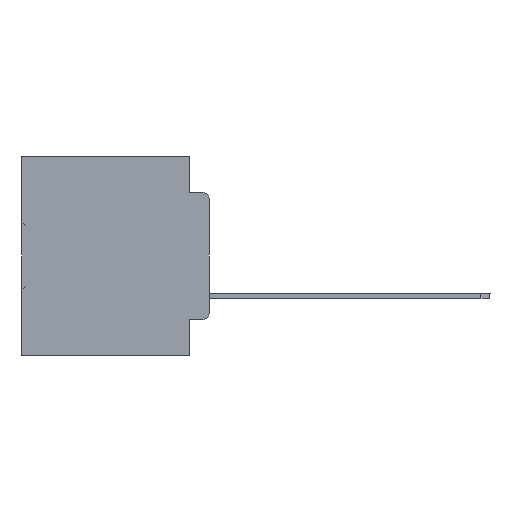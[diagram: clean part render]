
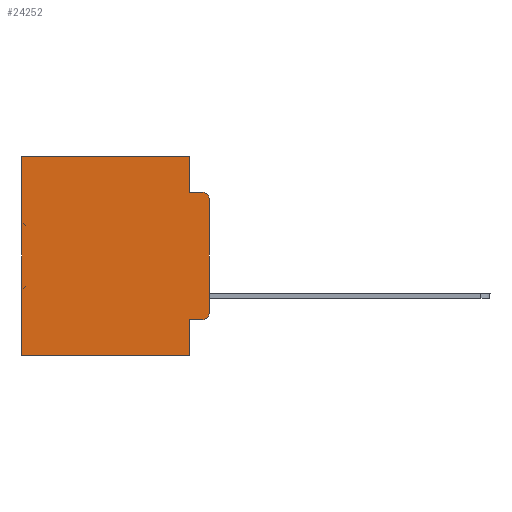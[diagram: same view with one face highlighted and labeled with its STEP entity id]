
A CAD part, left-side view. The second image highlights one B-rep face of the part: STEP entity #24252.
In plain terms, the highlighted planar face has unit normal (-1, 0, 0).
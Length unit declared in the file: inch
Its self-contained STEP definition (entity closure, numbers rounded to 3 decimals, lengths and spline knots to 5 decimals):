
#265 = DIRECTION ( 'NONE',  ( 0., 0., -1. ) ) ;
#486 = DIRECTION ( 'NONE',  ( 0., 1., 0. ) ) ;
#992 = ORIENTED_EDGE ( 'NONE', *, *, #2277, .T. ) ;
#1150 = CARTESIAN_POINT ( 'NONE',  ( 0.298, 0.02, -0.4115 ) ) ;
#1247 = CARTESIAN_POINT ( 'NONE',  ( 0.298, 0., -0.5 ) ) ;
#1260 = EDGE_CURVE ( 'NONE', #4417, #13636, #15243, .T. ) ;
#1427 = CARTESIAN_POINT ( 'NONE',  ( 0.298, 0.051, 0. ) ) ;
#1604 = ORIENTED_EDGE ( 'NONE', *, *, #29339, .F. ) ;
#1828 = ORIENTED_EDGE ( 'NONE', *, *, #32957, .T. ) ;
#1943 = CARTESIAN_POINT ( 'NONE',  ( 0.298, 0., -0.3915 ) ) ;
#2215 = CIRCLE ( 'NONE', #25763, 0.02 ) ;
#2277 = EDGE_CURVE ( 'NONE', #29301, #34442, #7477, .T. ) ;
#2846 = LINE ( 'NONE', #14070, #20878 ) ;
#3327 = CARTESIAN_POINT ( 'NONE',  ( 0.298, 0.051, -0.4115 ) ) ;
#3336 = DIRECTION ( 'NONE',  ( 0., 0., -1. ) ) ;
#3627 = VECTOR ( 'NONE', #486, 39.37008 ) ;
#4417 = VERTEX_POINT ( 'NONE', #9358 ) ;
#4768 = EDGE_CURVE ( 'NONE', #9812, #14329, #6210, .T. ) ;
#5054 = CARTESIAN_POINT ( 'NONE',  ( 0.298, 0.473, 0. ) ) ;
#6210 = LINE ( 'NONE', #36431, #3627 ) ;
#6419 = CARTESIAN_POINT ( 'NONE',  ( 0.298, 0.02, -0.0885 ) ) ;
#6586 = DIRECTION ( 'NONE',  ( 0., 0., -1. ) ) ;
#7319 = VERTEX_POINT ( 'NONE', #1943 ) ;
#7477 = CIRCLE ( 'NONE', #28071, 0.02 ) ;
#8354 = LINE ( 'NONE', #5054, #28795 ) ;
#9358 = CARTESIAN_POINT ( 'NONE',  ( 0.298, 0.051, -0.5 ) ) ;
#9449 = ORIENTED_EDGE ( 'NONE', *, *, #22322, .T. ) ;
#9744 = VECTOR ( 'NONE', #19666, 39.37008 ) ;
#9812 = VERTEX_POINT ( 'NONE', #30938 ) ;
#10072 = EDGE_CURVE ( 'NONE', #9812, #10567, #20572, .T. ) ;
#10567 = VERTEX_POINT ( 'NONE', #21561 ) ;
#11801 = DIRECTION ( 'NONE',  ( 1., 0., 0. ) ) ;
#13014 = AXIS2_PLACEMENT_3D ( 'NONE', #25818, #11801, #23044 ) ;
#13228 = VERTEX_POINT ( 'NONE', #3327 ) ;
#13515 = DIRECTION ( 'NONE',  ( 0., 0., -1. ) ) ;
#13636 = VERTEX_POINT ( 'NONE', #19661 ) ;
#13791 = EDGE_LOOP ( 'NONE', ( #1604, #992, #34383, #33699, #29240, #9449, #30137, #19341, #1828, #24848 ) ) ;
#14070 = CARTESIAN_POINT ( 'NONE',  ( 0.298, 0., 0. ) ) ;
#14329 = VERTEX_POINT ( 'NONE', #19032 ) ;
#14697 = CARTESIAN_POINT ( 'NONE',  ( 0.298, 0.051, 0. ) ) ;
#15243 = LINE ( 'NONE', #1247, #33209 ) ;
#15946 = DIRECTION ( 'NONE',  ( 0., 0., -1. ) ) ;
#17335 = DIRECTION ( 'NONE',  ( -1., 0., 0. ) ) ;
#18185 = LINE ( 'NONE', #1427, #21876 ) ;
#18336 = CARTESIAN_POINT ( 'NONE',  ( 0.298, 0.02, -0.3915 ) ) ;
#18686 = EDGE_CURVE ( 'NONE', #22680, #7319, #2215, .T. ) ;
#19032 = CARTESIAN_POINT ( 'NONE',  ( 0.298, 0.473, 0. ) ) ;
#19324 = VECTOR ( 'NONE', #31682, 39.37008 ) ;
#19341 = ORIENTED_EDGE ( 'NONE', *, *, #24824, .F. ) ;
#19661 = CARTESIAN_POINT ( 'NONE',  ( 0.298, 0.473, -0.5 ) ) ;
#19666 = DIRECTION ( 'NONE',  ( 0., -1., 0. ) ) ;
#19883 = EDGE_CURVE ( 'NONE', #10567, #34442, #34441, .T. ) ;
#20572 = LINE ( 'NONE', #14697, #27053 ) ;
#20878 = VECTOR ( 'NONE', #265, 39.37008 ) ;
#21561 = CARTESIAN_POINT ( 'NONE',  ( 0.298, 0.051, -0.0885 ) ) ;
#21876 = VECTOR ( 'NONE', #29428, 39.37008 ) ;
#22322 = EDGE_CURVE ( 'NONE', #14329, #13636, #8354, .T. ) ;
#22680 = VERTEX_POINT ( 'NONE', #1150 ) ;
#23044 = DIRECTION ( 'NONE',  ( 0., 0., -1. ) ) ;
#24252 = ADVANCED_FACE ( 'NONE', ( #31707 ), #25999, .F. ) ;
#24824 = EDGE_CURVE ( 'NONE', #13228, #4417, #18185, .T. ) ;
#24848 = ORIENTED_EDGE ( 'NONE', *, *, #18686, .T. ) ;
#25032 = LINE ( 'NONE', #33692, #9744 ) ;
#25248 = CARTESIAN_POINT ( 'NONE',  ( 0.298, 0.051, -0.0885 ) ) ;
#25763 = AXIS2_PLACEMENT_3D ( 'NONE', #18336, #29586, #15946 ) ;
#25818 = CARTESIAN_POINT ( 'NONE',  ( 0.298, 0., 0. ) ) ;
#25999 = PLANE ( 'NONE',  #13014 ) ;
#27053 = VECTOR ( 'NONE', #6586, 39.37008 ) ;
#28071 = AXIS2_PLACEMENT_3D ( 'NONE', #34284, #17335, #3336 ) ;
#28795 = VECTOR ( 'NONE', #13515, 39.37008 ) ;
#29240 = ORIENTED_EDGE ( 'NONE', *, *, #4768, .T. ) ;
#29301 = VERTEX_POINT ( 'NONE', #31235 ) ;
#29339 = EDGE_CURVE ( 'NONE', #29301, #7319, #2846, .T. ) ;
#29428 = DIRECTION ( 'NONE',  ( 0., 0., -1. ) ) ;
#29586 = DIRECTION ( 'NONE',  ( -1., 0., 0. ) ) ;
#30137 = ORIENTED_EDGE ( 'NONE', *, *, #1260, .F. ) ;
#30938 = CARTESIAN_POINT ( 'NONE',  ( 0.298, 0.051, 0. ) ) ;
#31235 = CARTESIAN_POINT ( 'NONE',  ( 0.298, 0., -0.1085 ) ) ;
#31682 = DIRECTION ( 'NONE',  ( 0., -1., 0. ) ) ;
#31707 = FACE_OUTER_BOUND ( 'NONE', #13791, .T. ) ;
#32216 = DIRECTION ( 'NONE',  ( 0., 1., 0. ) ) ;
#32957 = EDGE_CURVE ( 'NONE', #13228, #22680, #25032, .T. ) ;
#33209 = VECTOR ( 'NONE', #32216, 39.37008 ) ;
#33692 = CARTESIAN_POINT ( 'NONE',  ( 0.298, 0.051, -0.4115 ) ) ;
#33699 = ORIENTED_EDGE ( 'NONE', *, *, #10072, .F. ) ;
#34284 = CARTESIAN_POINT ( 'NONE',  ( 0.298, 0.02, -0.1085 ) ) ;
#34383 = ORIENTED_EDGE ( 'NONE', *, *, #19883, .F. ) ;
#34441 = LINE ( 'NONE', #25248, #19324 ) ;
#34442 = VERTEX_POINT ( 'NONE', #6419 ) ;
#36431 = CARTESIAN_POINT ( 'NONE',  ( 0.298, 0., 0. ) ) ;
